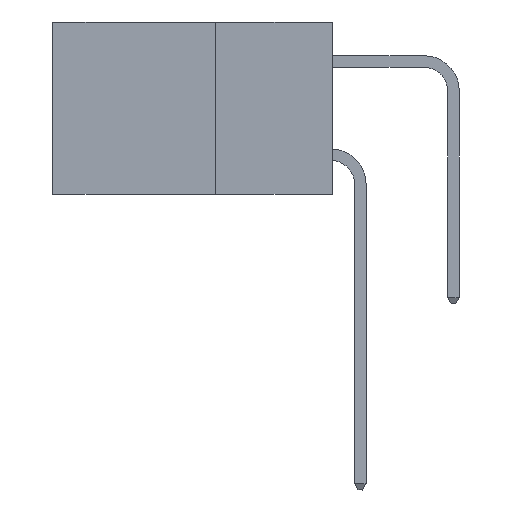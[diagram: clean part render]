
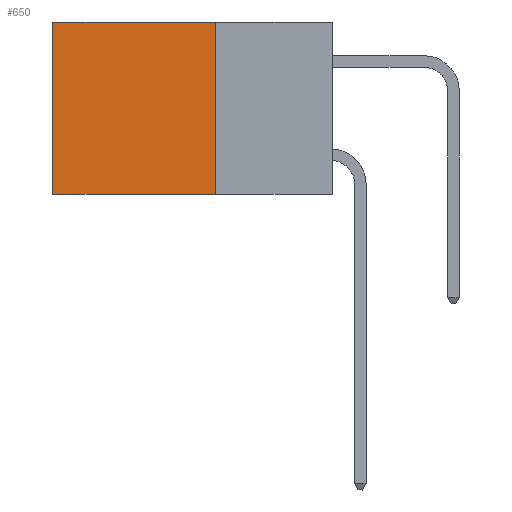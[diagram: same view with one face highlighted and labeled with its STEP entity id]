
A CAD part, left-side view. The second image highlights one B-rep face of the part: STEP entity #650.
In plain terms, the highlighted planar face has unit normal (-1, 0, 0).
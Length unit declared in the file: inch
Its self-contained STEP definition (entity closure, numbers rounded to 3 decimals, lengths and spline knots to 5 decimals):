
#287 = CARTESIAN_POINT ( 'NONE',  ( 0.298, 0.25, 0. ) ) ;
#376 = CARTESIAN_POINT ( 'NONE',  ( 0.298, 0.6, 0. ) ) ;
#650 = ADVANCED_FACE ( 'NONE', ( #11120 ), #1340, .F. ) ;
#1340 = PLANE ( 'NONE',  #2654 ) ;
#1382 = CARTESIAN_POINT ( 'NONE',  ( 0.298, 0.25, 0. ) ) ;
#1664 = EDGE_CURVE ( 'NONE', #5266, #3973, #5894, .T. ) ;
#1824 = VERTEX_POINT ( 'NONE', #8681 ) ;
#2654 = AXIS2_PLACEMENT_3D ( 'NONE', #7688, #8593, #6801 ) ;
#3892 = ORIENTED_EDGE ( 'NONE', *, *, #4662, .F. ) ;
#3897 = DIRECTION ( 'NONE',  ( 0., 1., 0. ) ) ;
#3973 = VERTEX_POINT ( 'NONE', #11087 ) ;
#4662 = EDGE_CURVE ( 'NONE', #7776, #3973, #10264, .T. ) ;
#4788 = VECTOR ( 'NONE', #9543, 39.37008 ) ;
#5266 = VERTEX_POINT ( 'NONE', #6027 ) ;
#5339 = ORIENTED_EDGE ( 'NONE', *, *, #6265, .T. ) ;
#5488 = LINE ( 'NONE', #1382, #4788 ) ;
#5557 = CARTESIAN_POINT ( 'NONE',  ( 0.298, 0.25, -0.37 ) ) ;
#5639 = ORIENTED_EDGE ( 'NONE', *, *, #6726, .F. ) ;
#5894 = LINE ( 'NONE', #376, #8323 ) ;
#6027 = CARTESIAN_POINT ( 'NONE',  ( 0.298, 0.6, 0. ) ) ;
#6265 = EDGE_CURVE ( 'NONE', #1824, #5266, #10375, .T. ) ;
#6726 = EDGE_CURVE ( 'NONE', #1824, #7776, #5488, .T. ) ;
#6801 = DIRECTION ( 'NONE',  ( 0., 0., -1. ) ) ;
#7688 = CARTESIAN_POINT ( 'NONE',  ( 0.298, 0.25, 0. ) ) ;
#7699 = DIRECTION ( 'NONE',  ( 0., 0., -1. ) ) ;
#7776 = VERTEX_POINT ( 'NONE', #10378 ) ;
#7853 = VECTOR ( 'NONE', #3897, 39.37008 ) ;
#7952 = VECTOR ( 'NONE', #9381, 39.37008 ) ;
#8323 = VECTOR ( 'NONE', #7699, 39.37008 ) ;
#8593 = DIRECTION ( 'NONE',  ( 1., 0., 0. ) ) ;
#8681 = CARTESIAN_POINT ( 'NONE',  ( 0.298, 0.25, 0. ) ) ;
#9315 = ORIENTED_EDGE ( 'NONE', *, *, #1664, .T. ) ;
#9381 = DIRECTION ( 'NONE',  ( 0., 1., 0. ) ) ;
#9543 = DIRECTION ( 'NONE',  ( 0., 0., -1. ) ) ;
#10264 = LINE ( 'NONE', #5557, #7853 ) ;
#10375 = LINE ( 'NONE', #287, #7952 ) ;
#10378 = CARTESIAN_POINT ( 'NONE',  ( 0.298, 0.25, -0.37 ) ) ;
#10907 = EDGE_LOOP ( 'NONE', ( #9315, #3892, #5639, #5339 ) ) ;
#11087 = CARTESIAN_POINT ( 'NONE',  ( 0.298, 0.6, -0.37 ) ) ;
#11120 = FACE_OUTER_BOUND ( 'NONE', #10907, .T. ) ;
